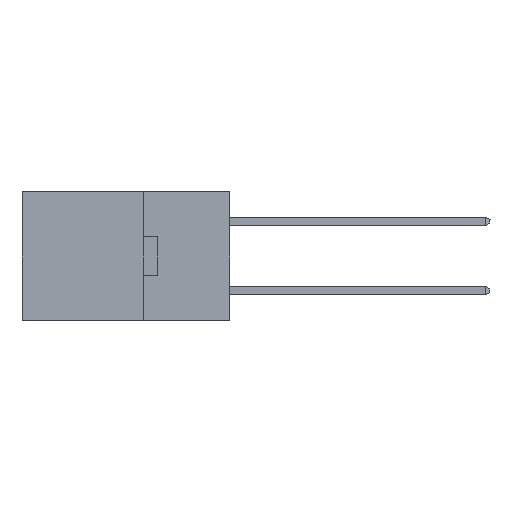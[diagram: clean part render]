
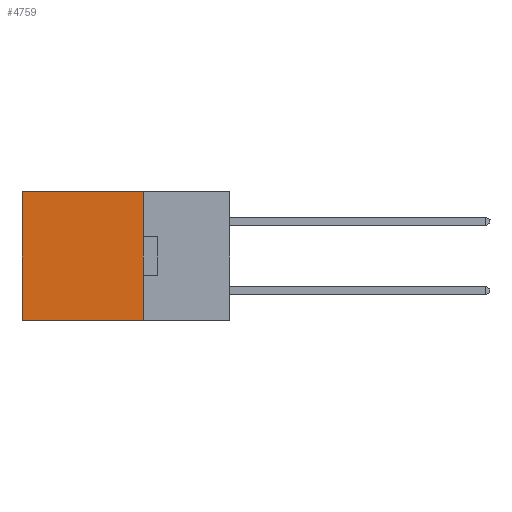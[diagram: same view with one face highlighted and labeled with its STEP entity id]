
A CAD part, left-side view. The second image highlights one B-rep face of the part: STEP entity #4759.
In plain terms, the highlighted planar face has unit normal (-1, 0, 0).
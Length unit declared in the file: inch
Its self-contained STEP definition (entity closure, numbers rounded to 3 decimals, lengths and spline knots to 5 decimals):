
#200 = EDGE_LOOP ( 'NONE', ( #18908, #9498, #8706, #10754 ) ) ;
#430 = CARTESIAN_POINT ( 'NONE',  ( 0.2615, 0.25, -0.37 ) ) ;
#916 = CARTESIAN_POINT ( 'NONE',  ( 0.2615, 0.25, -0.37 ) ) ;
#2684 = CARTESIAN_POINT ( 'NONE',  ( 0.2615, 0.25, -0.37 ) ) ;
#3097 = EDGE_CURVE ( 'NONE', #21540, #16541, #4889, .T. ) ;
#4634 = CARTESIAN_POINT ( 'NONE',  ( 0.2615, 0.6, 0. ) ) ;
#4759 = ADVANCED_FACE ( 'NONE', ( #13692 ), #11179, .F. ) ;
#4889 = LINE ( 'NONE', #13718, #24430 ) ;
#5039 = LINE ( 'NONE', #22292, #20276 ) ;
#5141 = DIRECTION ( 'NONE',  ( 1., 0., 0. ) ) ;
#5221 = VERTEX_POINT ( 'NONE', #5342 ) ;
#5342 = CARTESIAN_POINT ( 'NONE',  ( 0.2615, 0.6, -0.37 ) ) ;
#5809 = CARTESIAN_POINT ( 'NONE',  ( 0.2615, 0.25, 0. ) ) ;
#8706 = ORIENTED_EDGE ( 'NONE', *, *, #3097, .F. ) ;
#9082 = DIRECTION ( 'NONE',  ( 0., 0., -1. ) ) ;
#9374 = DIRECTION ( 'NONE',  ( 0., 0., -1. ) ) ;
#9498 = ORIENTED_EDGE ( 'NONE', *, *, #10846, .F. ) ;
#9556 = DIRECTION ( 'NONE',  ( 0., 1., 0. ) ) ;
#10754 = ORIENTED_EDGE ( 'NONE', *, *, #17710, .T. ) ;
#10844 = VECTOR ( 'NONE', #14088, 39.37008 ) ;
#10846 = EDGE_CURVE ( 'NONE', #16541, #5221, #20224, .T. ) ;
#11179 = PLANE ( 'NONE',  #25761 ) ;
#13692 = FACE_OUTER_BOUND ( 'NONE', #200, .T. ) ;
#13718 = CARTESIAN_POINT ( 'NONE',  ( 0.2615, 0.25, -0.37 ) ) ;
#14088 = DIRECTION ( 'NONE',  ( 0., 1., 0. ) ) ;
#16541 = VERTEX_POINT ( 'NONE', #2684 ) ;
#17363 = VECTOR ( 'NONE', #9556, 39.37008 ) ;
#17710 = EDGE_CURVE ( 'NONE', #21540, #18582, #25027, .T. ) ;
#18582 = VERTEX_POINT ( 'NONE', #4634 ) ;
#18908 = ORIENTED_EDGE ( 'NONE', *, *, #27538, .T. ) ;
#20171 = DIRECTION ( 'NONE',  ( 0., 0., -1. ) ) ;
#20224 = LINE ( 'NONE', #430, #17363 ) ;
#20276 = VECTOR ( 'NONE', #9374, 39.37008 ) ;
#21540 = VERTEX_POINT ( 'NONE', #21821 ) ;
#21821 = CARTESIAN_POINT ( 'NONE',  ( 0.2615, 0.25, 0. ) ) ;
#22292 = CARTESIAN_POINT ( 'NONE',  ( 0.2615, 0.6, -0.37 ) ) ;
#24430 = VECTOR ( 'NONE', #20171, 39.37008 ) ;
#25027 = LINE ( 'NONE', #5809, #10844 ) ;
#25761 = AXIS2_PLACEMENT_3D ( 'NONE', #916, #5141, #9082 ) ;
#27538 = EDGE_CURVE ( 'NONE', #18582, #5221, #5039, .T. ) ;
